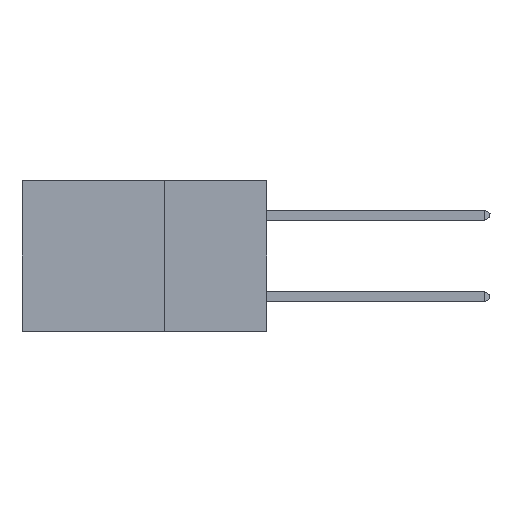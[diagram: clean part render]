
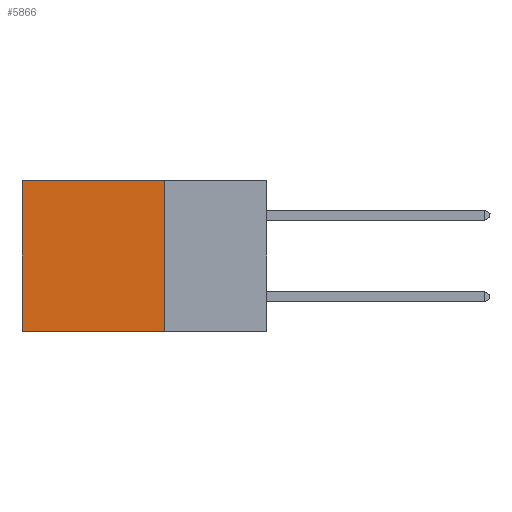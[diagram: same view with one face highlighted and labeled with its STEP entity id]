
A CAD part, left-side view. The second image highlights one B-rep face of the part: STEP entity #5866.
In plain terms, the highlighted planar face has unit normal (-1, 0, 0).
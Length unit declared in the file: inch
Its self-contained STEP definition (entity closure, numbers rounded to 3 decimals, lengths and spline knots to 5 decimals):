
#358 = CARTESIAN_POINT ( 'NONE',  ( 0.2875, 0.6, 0. ) ) ;
#945 = CARTESIAN_POINT ( 'NONE',  ( 0.2875, 0.25, -0.37 ) ) ;
#1379 = DIRECTION ( 'NONE',  ( 0., 1., 0. ) ) ;
#1388 = VECTOR ( 'NONE', #1636, 39.37008 ) ;
#1636 = DIRECTION ( 'NONE',  ( 0., 0., -1. ) ) ;
#1833 = EDGE_CURVE ( 'NONE', #7425, #11138, #4690, .T. ) ;
#1879 = FACE_OUTER_BOUND ( 'NONE', #11812, .T. ) ;
#2329 = EDGE_CURVE ( 'NONE', #7129, #11138, #13061, .T. ) ;
#2345 = DIRECTION ( 'NONE',  ( 1., 0., 0. ) ) ;
#3097 = VECTOR ( 'NONE', #1379, 39.37008 ) ;
#4690 = LINE ( 'NONE', #6599, #1388 ) ;
#5452 = CARTESIAN_POINT ( 'NONE',  ( 0.2875, 0.25, 0. ) ) ;
#5545 = DIRECTION ( 'NONE',  ( 0., 0., -1. ) ) ;
#5800 = VECTOR ( 'NONE', #7586, 39.37008 ) ;
#5866 = ADVANCED_FACE ( 'NONE', ( #1879 ), #8700, .F. ) ;
#5915 = LINE ( 'NONE', #8860, #3097 ) ;
#6599 = CARTESIAN_POINT ( 'NONE',  ( 0.2875, 0.6, 0. ) ) ;
#6617 = EDGE_CURVE ( 'NONE', #9181, #7425, #5915, .T. ) ;
#7129 = VERTEX_POINT ( 'NONE', #945 ) ;
#7425 = VERTEX_POINT ( 'NONE', #358 ) ;
#7473 = VECTOR ( 'NONE', #5545, 39.37008 ) ;
#7586 = DIRECTION ( 'NONE',  ( 0., 1., 0. ) ) ;
#7672 = CARTESIAN_POINT ( 'NONE',  ( 0.2875, 0.25, -0.37 ) ) ;
#7911 = ORIENTED_EDGE ( 'NONE', *, *, #1833, .T. ) ;
#7937 = ORIENTED_EDGE ( 'NONE', *, *, #2329, .F. ) ;
#7975 = ORIENTED_EDGE ( 'NONE', *, *, #10918, .F. ) ;
#7986 = ORIENTED_EDGE ( 'NONE', *, *, #6617, .T. ) ;
#8700 = PLANE ( 'NONE',  #9102 ) ;
#8860 = CARTESIAN_POINT ( 'NONE',  ( 0.2875, 0.25, 0. ) ) ;
#8899 = CARTESIAN_POINT ( 'NONE',  ( 0.2875, 0.6, -0.37 ) ) ;
#9102 = AXIS2_PLACEMENT_3D ( 'NONE', #13407, #2345, #9690 ) ;
#9181 = VERTEX_POINT ( 'NONE', #12574 ) ;
#9690 = DIRECTION ( 'NONE',  ( 0., 0., -1. ) ) ;
#10125 = LINE ( 'NONE', #5452, #7473 ) ;
#10918 = EDGE_CURVE ( 'NONE', #9181, #7129, #10125, .T. ) ;
#11138 = VERTEX_POINT ( 'NONE', #8899 ) ;
#11812 = EDGE_LOOP ( 'NONE', ( #7911, #7937, #7975, #7986 ) ) ;
#12574 = CARTESIAN_POINT ( 'NONE',  ( 0.2875, 0.25, 0. ) ) ;
#13061 = LINE ( 'NONE', #7672, #5800 ) ;
#13407 = CARTESIAN_POINT ( 'NONE',  ( 0.2875, 0.25, 0. ) ) ;
